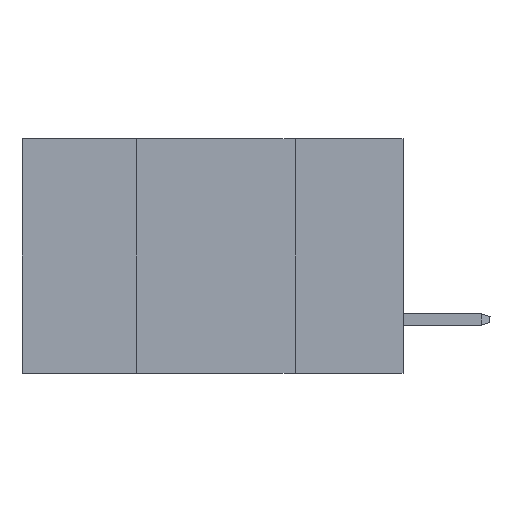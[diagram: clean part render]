
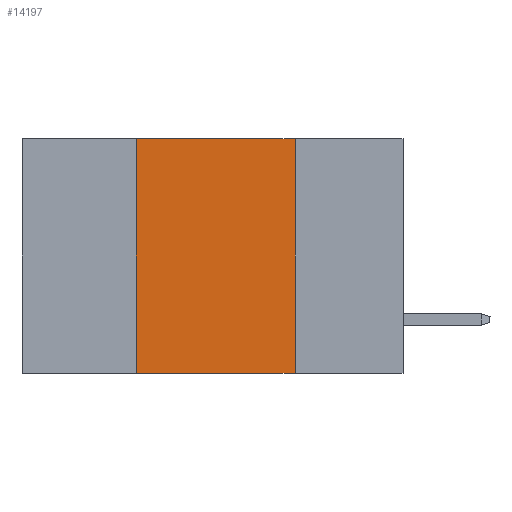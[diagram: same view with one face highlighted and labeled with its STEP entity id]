
A CAD part, left-side view. The second image highlights one B-rep face of the part: STEP entity #14197.
In plain terms, the highlighted planar face has unit normal (-1, 0, 0).
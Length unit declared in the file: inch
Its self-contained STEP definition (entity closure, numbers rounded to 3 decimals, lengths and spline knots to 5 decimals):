
#726 = ORIENTED_EDGE ( 'NONE', *, *, #6861, .F. ) ;
#1176 = CARTESIAN_POINT ( 'NONE',  ( 0., 0.6, 0. ) ) ;
#1823 = VERTEX_POINT ( 'NONE', #13283 ) ;
#1973 = CARTESIAN_POINT ( 'NONE',  ( 0., 0.17, -0.37 ) ) ;
#2105 = CARTESIAN_POINT ( 'NONE',  ( 0., 0.6, -0.37 ) ) ;
#2945 = AXIS2_PLACEMENT_3D ( 'NONE', #5366, #10010, #3061 ) ;
#3061 = DIRECTION ( 'NONE',  ( 0., 0., -1. ) ) ;
#3923 = EDGE_CURVE ( 'NONE', #5085, #10291, #6777, .T. ) ;
#3976 = VECTOR ( 'NONE', #8398, 39.37008 ) ;
#4007 = CARTESIAN_POINT ( 'NONE',  ( 0., 0.42, 0. ) ) ;
#4084 = LINE ( 'NONE', #10186, #12338 ) ;
#5000 = ORIENTED_EDGE ( 'NONE', *, *, #9274, .F. ) ;
#5016 = DIRECTION ( 'NONE',  ( 0., 0., 1. ) ) ;
#5085 = VERTEX_POINT ( 'NONE', #5749 ) ;
#5366 = CARTESIAN_POINT ( 'NONE',  ( 0., 0.6, 0. ) ) ;
#5749 = CARTESIAN_POINT ( 'NONE',  ( 0., 0.42, -0.37 ) ) ;
#6519 = PLANE ( 'NONE',  #2945 ) ;
#6777 = LINE ( 'NONE', #2105, #11269 ) ;
#6861 = EDGE_CURVE ( 'NONE', #7450, #1823, #10583, .T. ) ;
#7450 = VERTEX_POINT ( 'NONE', #4007 ) ;
#8100 = ORIENTED_EDGE ( 'NONE', *, *, #3923, .T. ) ;
#8271 = EDGE_LOOP ( 'NONE', ( #5000, #726, #12249, #8100 ) ) ;
#8398 = DIRECTION ( 'NONE',  ( 0., -1., 0. ) ) ;
#9274 = EDGE_CURVE ( 'NONE', #1823, #10291, #4084, .T. ) ;
#10010 = DIRECTION ( 'NONE',  ( 1., 0., 0. ) ) ;
#10186 = CARTESIAN_POINT ( 'NONE',  ( 0., 0.17, 0. ) ) ;
#10291 = VERTEX_POINT ( 'NONE', #1973 ) ;
#10564 = EDGE_CURVE ( 'NONE', #5085, #7450, #14706, .T. ) ;
#10583 = LINE ( 'NONE', #1176, #3976 ) ;
#11269 = VECTOR ( 'NONE', #11495, 39.37008 ) ;
#11495 = DIRECTION ( 'NONE',  ( 0., -1., 0. ) ) ;
#12249 = ORIENTED_EDGE ( 'NONE', *, *, #10564, .F. ) ;
#12336 = VECTOR ( 'NONE', #5016, 39.37008 ) ;
#12338 = VECTOR ( 'NONE', #12378, 39.37008 ) ;
#12378 = DIRECTION ( 'NONE',  ( 0., 0., -1. ) ) ;
#12510 = FACE_OUTER_BOUND ( 'NONE', #8271, .T. ) ;
#13283 = CARTESIAN_POINT ( 'NONE',  ( 0., 0.17, 0. ) ) ;
#13310 = CARTESIAN_POINT ( 'NONE',  ( 0., 0.42, 0. ) ) ;
#14197 = ADVANCED_FACE ( 'NONE', ( #12510 ), #6519, .F. ) ;
#14706 = LINE ( 'NONE', #13310, #12336 ) ;
